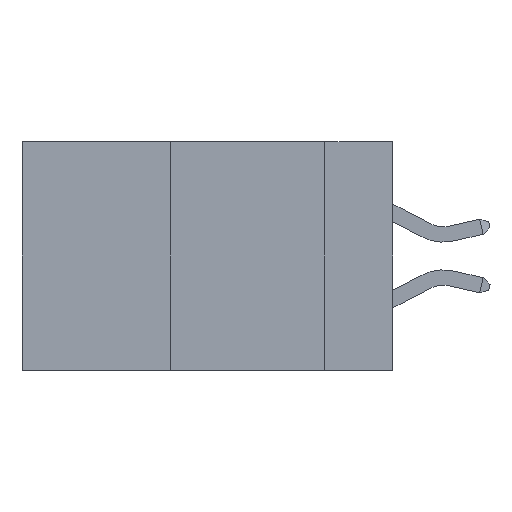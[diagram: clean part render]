
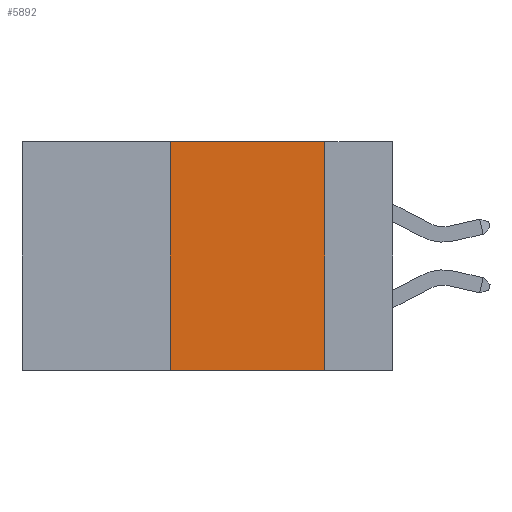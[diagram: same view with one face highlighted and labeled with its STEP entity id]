
A CAD part, left-side view. The second image highlights one B-rep face of the part: STEP entity #5892.
In plain terms, the highlighted planar face has unit normal (-1, 0, 0).
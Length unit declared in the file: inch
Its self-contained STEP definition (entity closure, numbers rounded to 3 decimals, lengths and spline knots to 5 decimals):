
#647 = VECTOR ( 'NONE', #11689, 39.37008 ) ;
#1227 = EDGE_LOOP ( 'NONE', ( #19199, #5851, #11002, #14866 ) ) ;
#2504 = CARTESIAN_POINT ( 'NONE',  ( 0., 0.6, -0.37 ) ) ;
#3727 = EDGE_CURVE ( 'NONE', #20896, #4147, #14517, .T. ) ;
#4147 = VERTEX_POINT ( 'NONE', #17274 ) ;
#4340 = LINE ( 'NONE', #17808, #21790 ) ;
#5771 = DIRECTION ( 'NONE',  ( 1., 0., 0. ) ) ;
#5851 = ORIENTED_EDGE ( 'NONE', *, *, #17580, .F. ) ;
#5892 = ADVANCED_FACE ( 'NONE', ( #12035 ), #15256, .F. ) ;
#6555 = CARTESIAN_POINT ( 'NONE',  ( 0., 0.6, 0. ) ) ;
#7616 = VECTOR ( 'NONE', #16699, 39.37008 ) ;
#7671 = DIRECTION ( 'NONE',  ( 0., 0., 1. ) ) ;
#7862 = EDGE_CURVE ( 'NONE', #20896, #18555, #4340, .T. ) ;
#8130 = LINE ( 'NONE', #22163, #16620 ) ;
#10940 = CARTESIAN_POINT ( 'NONE',  ( 0., 0.36, 0. ) ) ;
#11002 = ORIENTED_EDGE ( 'NONE', *, *, #7862, .F. ) ;
#11689 = DIRECTION ( 'NONE',  ( 0., -1., 0. ) ) ;
#12035 = FACE_OUTER_BOUND ( 'NONE', #1227, .T. ) ;
#12036 = DIRECTION ( 'NONE',  ( 0., 0., -1. ) ) ;
#12140 = CARTESIAN_POINT ( 'NONE',  ( 0., 0.6, 0. ) ) ;
#12269 = CARTESIAN_POINT ( 'NONE',  ( 0., 0.36, -0.37 ) ) ;
#13131 = EDGE_CURVE ( 'NONE', #20666, #4147, #8130, .T. ) ;
#14374 = AXIS2_PLACEMENT_3D ( 'NONE', #12140, #5771, #12036 ) ;
#14517 = LINE ( 'NONE', #2504, #647 ) ;
#14866 = ORIENTED_EDGE ( 'NONE', *, *, #3727, .T. ) ;
#15256 = PLANE ( 'NONE',  #14374 ) ;
#16620 = VECTOR ( 'NONE', #17258, 39.37008 ) ;
#16699 = DIRECTION ( 'NONE',  ( 0., -1., 0. ) ) ;
#17163 = LINE ( 'NONE', #6555, #7616 ) ;
#17258 = DIRECTION ( 'NONE',  ( 0., 0., -1. ) ) ;
#17274 = CARTESIAN_POINT ( 'NONE',  ( 0., 0.11, -0.37 ) ) ;
#17580 = EDGE_CURVE ( 'NONE', #18555, #20666, #17163, .T. ) ;
#17808 = CARTESIAN_POINT ( 'NONE',  ( 0., 0.36, 0. ) ) ;
#18555 = VERTEX_POINT ( 'NONE', #10940 ) ;
#19199 = ORIENTED_EDGE ( 'NONE', *, *, #13131, .F. ) ;
#20036 = CARTESIAN_POINT ( 'NONE',  ( 0., 0.11, 0. ) ) ;
#20666 = VERTEX_POINT ( 'NONE', #20036 ) ;
#20896 = VERTEX_POINT ( 'NONE', #12269 ) ;
#21790 = VECTOR ( 'NONE', #7671, 39.37008 ) ;
#22163 = CARTESIAN_POINT ( 'NONE',  ( 0., 0.11, 0. ) ) ;
